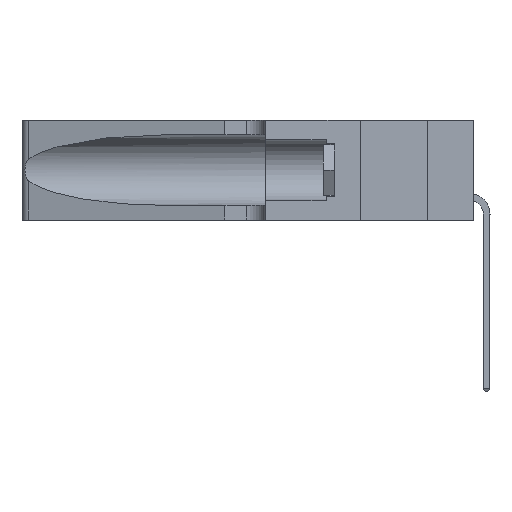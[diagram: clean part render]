
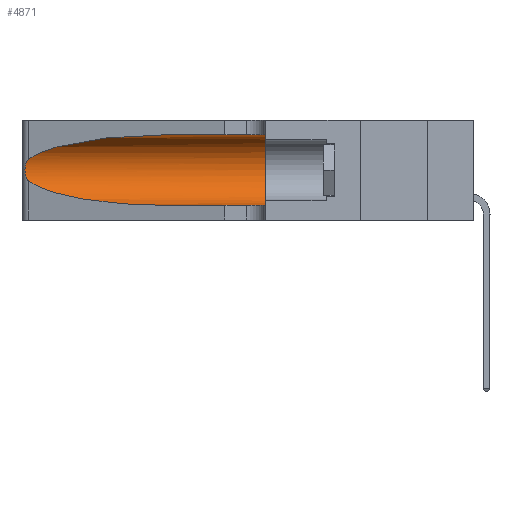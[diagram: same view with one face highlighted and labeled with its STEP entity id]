
A CAD part, left-side view. The second image highlights one B-rep face of the part: STEP entity #4871.
In plain terms, the highlighted cylindrical face has radius 3.308 mm (diameter 6.617 mm), a partial arc.
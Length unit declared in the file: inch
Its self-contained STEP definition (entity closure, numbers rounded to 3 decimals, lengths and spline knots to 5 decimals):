
#17 = VERTEX_POINT ( 'NONE', #14931 ) ;
#44 =( BOUNDED_CURVE ( )  B_SPLINE_CURVE ( 3, ( #9845, #705, #11447, #868 ),
 .UNSPECIFIED., .F., .T. ) 
 B_SPLINE_CURVE_WITH_KNOTS ( ( 4, 4 ),
 ( 1.5708, 2.84003 ),
 .UNSPECIFIED. ) 
 CURVE ( )  GEOMETRIC_REPRESENTATION_ITEM ( )  RATIONAL_B_SPLINE_CURVE ( ( 1., 0.87, 0.87, 1. ) ) 
 REPRESENTATION_ITEM ( '' )  );
#330 = CYLINDRICAL_SURFACE ( 'NONE', #4571, 0.13025 ) ;
#705 = CARTESIAN_POINT ( 'NONE',  ( 0.18966, 0.96281, 0.31525 ) ) ;
#775 = CARTESIAN_POINT ( 'NONE',  ( 0.25787, 1.23484, 0.2124 ) ) ;
#789 = B_SPLINE_CURVE_WITH_KNOTS ( 'NONE', 3,
 ( #4175, #20115, #21977, #775, #6093, #7893, #20183, #11437, #6764, #6681, #19078, #12149, #20607, #22554 ),
 .UNSPECIFIED., .F., .F.,
 ( 4, 2, 2, 2, 2, 2, 4 ),
 ( 0., 0.00027, 0.00053, 0.00107, 0.0016, 0.00187, 0.00214 ),
 .UNSPECIFIED. ) ;
#868 = CARTESIAN_POINT ( 'NONE',  ( 0.25487, 1.22718, 0.22369 ) ) ;
#1338 = ORIENTED_EDGE ( 'NONE', *, *, #20422, .T. ) ;
#2105 = CIRCLE ( 'NONE', #10251, 0.13025 ) ;
#2938 = VECTOR ( 'NONE', #11924, 39.37008 ) ;
#4175 = CARTESIAN_POINT ( 'NONE',  ( 0.25487, 1.22718, 0.22369 ) ) ;
#4188 =( BOUNDED_CURVE ( )  B_SPLINE_CURVE ( 3, ( #19306, #10567, #21006, #14154 ),
 .UNSPECIFIED., .F., .F. ) 
 B_SPLINE_CURVE_WITH_KNOTS ( ( 4, 4 ),
 ( 3.44316, 4.71239 ),
 .UNSPECIFIED. ) 
 CURVE ( )  GEOMETRIC_REPRESENTATION_ITEM ( )  RATIONAL_B_SPLINE_CURVE ( ( 1., 0.87, 0.87, 1. ) ) 
 REPRESENTATION_ITEM ( '' )  );
#4571 = AXIS2_PLACEMENT_3D ( 'NONE', #4954, #6743, #8533 ) ;
#4864 = LINE ( 'NONE', #17098, #2938 ) ;
#4871 = ADVANCED_FACE ( 'NONE', ( #6715 ), #330, .F. ) ;
#4948 = CARTESIAN_POINT ( 'NONE',  ( 0.1305, 0.35, 0.05475 ) ) ;
#4954 = CARTESIAN_POINT ( 'NONE',  ( 0.1305, 1.61858, 0.185 ) ) ;
#5497 = VERTEX_POINT ( 'NONE', #9286 ) ;
#6093 = CARTESIAN_POINT ( 'NONE',  ( 0.25854, 1.2359, 0.20912 ) ) ;
#6681 = CARTESIAN_POINT ( 'NONE',  ( 0.25856, 1.23593, 0.16098 ) ) ;
#6715 = FACE_OUTER_BOUND ( 'NONE', #7125, .T. ) ;
#6743 = DIRECTION ( 'NONE',  ( 0., -1., 0. ) ) ;
#6764 = CARTESIAN_POINT ( 'NONE',  ( 0.26017, 1.23833, 0.17102 ) ) ;
#6953 = DIRECTION ( 'NONE',  ( 0., -1., 0. ) ) ;
#7125 = EDGE_LOOP ( 'NONE', ( #1338, #11701, #20888, #10624, #15376, #9061 ) ) ;
#7893 = CARTESIAN_POINT ( 'NONE',  ( 0.26018, 1.23835, 0.19895 ) ) ;
#8533 = DIRECTION ( 'NONE',  ( 0., 0., -1. ) ) ;
#8837 = CARTESIAN_POINT ( 'NONE',  ( 0.1305, 0.35, 0.185 ) ) ;
#8952 = EDGE_CURVE ( 'NONE', #5497, #15848, #4864, .T. ) ;
#9000 = DIRECTION ( 'NONE',  ( 0., 0., 1. ) ) ;
#9061 = ORIENTED_EDGE ( 'NONE', *, *, #8952, .F. ) ;
#9286 = CARTESIAN_POINT ( 'NONE',  ( 0.1305, 0.72297, 0.31525 ) ) ;
#9400 = VECTOR ( 'NONE', #6953, 39.37008 ) ;
#9845 = CARTESIAN_POINT ( 'NONE',  ( 0.1305, 0.72297, 0.31525 ) ) ;
#10251 = AXIS2_PLACEMENT_3D ( 'NONE', #8837, #21217, #9000 ) ;
#10567 = CARTESIAN_POINT ( 'NONE',  ( 0.2373, 1.15595, 0.08982 ) ) ;
#10624 = ORIENTED_EDGE ( 'NONE', *, *, #13706, .T. ) ;
#11437 = CARTESIAN_POINT ( 'NONE',  ( 0.26075, 1.23896, 0.178 ) ) ;
#11447 = CARTESIAN_POINT ( 'NONE',  ( 0.2373, 1.15595, 0.28018 ) ) ;
#11701 = ORIENTED_EDGE ( 'NONE', *, *, #19442, .T. ) ;
#11924 = DIRECTION ( 'NONE',  ( 0., -1., 0. ) ) ;
#12149 = CARTESIAN_POINT ( 'NONE',  ( 0.25639, 1.23186, 0.15144 ) ) ;
#12255 = CARTESIAN_POINT ( 'NONE',  ( 0.1305, 0.72297, 0.05475 ) ) ;
#13706 = EDGE_CURVE ( 'NONE', #15625, #18996, #20927, .T. ) ;
#14154 = CARTESIAN_POINT ( 'NONE',  ( 0.1305, 0.72297, 0.05475 ) ) ;
#14931 = CARTESIAN_POINT ( 'NONE',  ( 0.25487, 1.22718, 0.14631 ) ) ;
#15376 = ORIENTED_EDGE ( 'NONE', *, *, #20210, .F. ) ;
#15625 = VERTEX_POINT ( 'NONE', #12255 ) ;
#15848 = VERTEX_POINT ( 'NONE', #19150 ) ;
#16961 = VERTEX_POINT ( 'NONE', #19471 ) ;
#17098 = CARTESIAN_POINT ( 'NONE',  ( 0.1305, 1.61858, 0.31525 ) ) ;
#18996 = VERTEX_POINT ( 'NONE', #4948 ) ;
#19078 = CARTESIAN_POINT ( 'NONE',  ( 0.25789, 1.23486, 0.15765 ) ) ;
#19150 = CARTESIAN_POINT ( 'NONE',  ( 0.1305, 0.35, 0.31525 ) ) ;
#19166 = CARTESIAN_POINT ( 'NONE',  ( 0.1305, 1.61858, 0.05475 ) ) ;
#19306 = CARTESIAN_POINT ( 'NONE',  ( 0.25487, 1.22718, 0.14631 ) ) ;
#19442 = EDGE_CURVE ( 'NONE', #16961, #17, #789, .T. ) ;
#19471 = CARTESIAN_POINT ( 'NONE',  ( 0.25487, 1.22718, 0.22369 ) ) ;
#20115 = CARTESIAN_POINT ( 'NONE',  ( 0.25555, 1.22994, 0.2215 ) ) ;
#20183 = CARTESIAN_POINT ( 'NONE',  ( 0.26075, 1.23896, 0.19203 ) ) ;
#20210 = EDGE_CURVE ( 'NONE', #15848, #18996, #2105, .T. ) ;
#20422 = EDGE_CURVE ( 'NONE', #5497, #16961, #44, .T. ) ;
#20607 = CARTESIAN_POINT ( 'NONE',  ( 0.25555, 1.22993, 0.14849 ) ) ;
#20888 = ORIENTED_EDGE ( 'NONE', *, *, #22418, .T. ) ;
#20927 = LINE ( 'NONE', #19166, #9400 ) ;
#21006 = CARTESIAN_POINT ( 'NONE',  ( 0.18966, 0.96281, 0.05475 ) ) ;
#21217 = DIRECTION ( 'NONE',  ( 0., 1., 0. ) ) ;
#21977 = CARTESIAN_POINT ( 'NONE',  ( 0.25639, 1.23184, 0.21858 ) ) ;
#22418 = EDGE_CURVE ( 'NONE', #17, #15625, #4188, .T. ) ;
#22554 = CARTESIAN_POINT ( 'NONE',  ( 0.25487, 1.22718, 0.14631 ) ) ;
